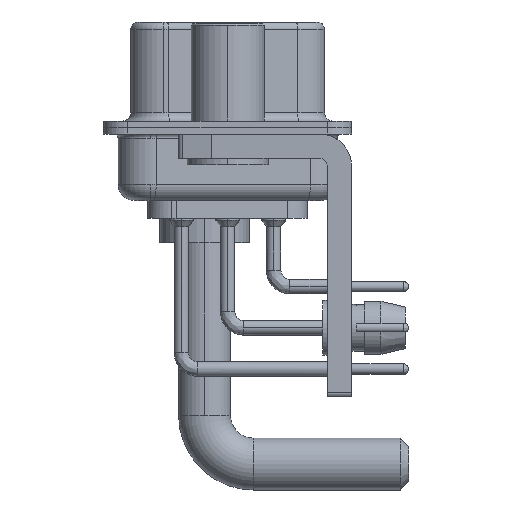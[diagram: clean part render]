
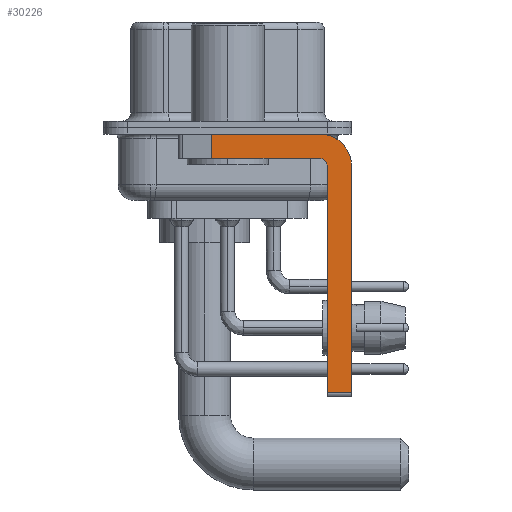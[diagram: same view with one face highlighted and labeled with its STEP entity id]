
A CAD part, left-side view. The second image highlights one B-rep face of the part: STEP entity #30226.
In plain terms, the highlighted planar face has unit normal (-1, 0, 0).
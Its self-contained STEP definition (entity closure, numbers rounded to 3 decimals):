
#754 = CIRCLE ( 'NONE', #32873, 2. ) ;
#1200 = DIRECTION ( 'NONE',  ( 0., -1., 0. ) ) ;
#2217 = AXIS2_PLACEMENT_3D ( 'NONE', #25078, #24886, #34525 ) ;
#3207 = VERTEX_POINT ( 'NONE', #11992 ) ;
#3504 = CIRCLE ( 'NONE', #2217, 0.5 ) ;
#3654 = CARTESIAN_POINT ( 'NONE',  ( -2.9, -6.15, -16.35 ) ) ;
#3787 = LINE ( 'NONE', #34758, #17340 ) ;
#4307 = VERTEX_POINT ( 'NONE', #29356 ) ;
#4416 = CARTESIAN_POINT ( 'NONE',  ( -2.9, -6.15, -2.4 ) ) ;
#4667 = VECTOR ( 'NONE', #13825, 1000. ) ;
#7042 = VERTEX_POINT ( 'NONE', #23971 ) ;
#7475 = ORIENTED_EDGE ( 'NONE', *, *, #37655, .F. ) ;
#8603 = DIRECTION ( 'NONE',  ( 0., 0., -1. ) ) ;
#8733 = CARTESIAN_POINT ( 'NONE',  ( -2.9, -5.65, -1.9 ) ) ;
#8794 = ORIENTED_EDGE ( 'NONE', *, *, #25865, .F. ) ;
#10162 = CARTESIAN_POINT ( 'NONE',  ( -2.9, -5.65, -0.4 ) ) ;
#11988 = ORIENTED_EDGE ( 'NONE', *, *, #27768, .F. ) ;
#11992 = CARTESIAN_POINT ( 'NONE',  ( -2.9, 0.978, -1.9 ) ) ;
#12527 = EDGE_CURVE ( 'NONE', #19139, #35585, #754, .T. ) ;
#12539 = VERTEX_POINT ( 'NONE', #3654 ) ;
#12830 = ORIENTED_EDGE ( 'NONE', *, *, #20391, .T. ) ;
#13825 = DIRECTION ( 'NONE',  ( 0., 1., 0. ) ) ;
#15504 = EDGE_CURVE ( 'NONE', #7042, #3207, #34600, .T. ) ;
#16035 = DIRECTION ( 'NONE',  ( 0., 0., -1. ) ) ;
#16162 = ORIENTED_EDGE ( 'NONE', *, *, #30370, .F. ) ;
#16312 = CARTESIAN_POINT ( 'NONE',  ( -2.9, -5.65, -2.4 ) ) ;
#16370 = VECTOR ( 'NONE', #39001, 1000. ) ;
#17340 = VECTOR ( 'NONE', #16035, 1000. ) ;
#17627 = AXIS2_PLACEMENT_3D ( 'NONE', #38975, #27314, #8603 ) ;
#17669 = DIRECTION ( 'NONE',  ( 0., -1., 0. ) ) ;
#17822 = LINE ( 'NONE', #30131, #29664 ) ;
#17860 = CARTESIAN_POINT ( 'NONE',  ( -2.9, 3., -0.4 ) ) ;
#18725 = ORIENTED_EDGE ( 'NONE', *, *, #15504, .T. ) ;
#19075 = VECTOR ( 'NONE', #1200, 1000. ) ;
#19139 = VERTEX_POINT ( 'NONE', #10162 ) ;
#20391 = EDGE_CURVE ( 'NONE', #12539, #4307, #31024, .T. ) ;
#21057 = FACE_OUTER_BOUND ( 'NONE', #24757, .T. ) ;
#22909 = CARTESIAN_POINT ( 'NONE',  ( -2.9, -5.65, -1.9 ) ) ;
#23730 = LINE ( 'NONE', #17860, #30975 ) ;
#23971 = CARTESIAN_POINT ( 'NONE',  ( -2.9, 0.978, -0.4 ) ) ;
#24103 = PLANE ( 'NONE',  #17627 ) ;
#24757 = EDGE_LOOP ( 'NONE', ( #11988, #18725, #7475, #16162, #8794, #12830, #38616, #29473 ) ) ;
#24886 = DIRECTION ( 'NONE',  ( -1., 0., 0. ) ) ;
#25078 = CARTESIAN_POINT ( 'NONE',  ( -2.9, -5.65, -2.4 ) ) ;
#25563 = CARTESIAN_POINT ( 'NONE',  ( -2.9, -7.65, -2.4 ) ) ;
#25865 = EDGE_CURVE ( 'NONE', #12539, #35719, #17822, .T. ) ;
#27306 = DIRECTION ( 'NONE',  ( 0., 0., 1. ) ) ;
#27314 = DIRECTION ( 'NONE',  ( 1., 0., 0. ) ) ;
#27768 = EDGE_CURVE ( 'NONE', #7042, #19139, #23730, .T. ) ;
#28514 = VERTEX_POINT ( 'NONE', #8733 ) ;
#29150 = LINE ( 'NONE', #22909, #4667 ) ;
#29356 = CARTESIAN_POINT ( 'NONE',  ( -2.9, -7.65, -16.35 ) ) ;
#29473 = ORIENTED_EDGE ( 'NONE', *, *, #12527, .F. ) ;
#29664 = VECTOR ( 'NONE', #27306, 1000. ) ;
#30131 = CARTESIAN_POINT ( 'NONE',  ( -2.9, -6.15, -16.6 ) ) ;
#30226 = ADVANCED_FACE ( 'NONE', ( #21057 ), #24103, .F. ) ;
#30370 = EDGE_CURVE ( 'NONE', #35719, #28514, #3504, .T. ) ;
#30975 = VECTOR ( 'NONE', #17669, 1000. ) ;
#31024 = LINE ( 'NONE', #37219, #19075 ) ;
#31239 = DIRECTION ( 'NONE',  ( 0., 0., -1. ) ) ;
#31595 = CARTESIAN_POINT ( 'NONE',  ( -2.9, 0.978, -1.9 ) ) ;
#32873 = AXIS2_PLACEMENT_3D ( 'NONE', #16312, #34236, #31239 ) ;
#34236 = DIRECTION ( 'NONE',  ( 1., 0., 0. ) ) ;
#34289 = EDGE_CURVE ( 'NONE', #35585, #4307, #3787, .T. ) ;
#34525 = DIRECTION ( 'NONE',  ( 0., 0., 1. ) ) ;
#34600 = LINE ( 'NONE', #31595, #16370 ) ;
#34758 = CARTESIAN_POINT ( 'NONE',  ( -2.9, -7.65, -2.4 ) ) ;
#35585 = VERTEX_POINT ( 'NONE', #25563 ) ;
#35719 = VERTEX_POINT ( 'NONE', #4416 ) ;
#37219 = CARTESIAN_POINT ( 'NONE',  ( -2.9, -5.65, -16.35 ) ) ;
#37655 = EDGE_CURVE ( 'NONE', #28514, #3207, #29150, .T. ) ;
#38616 = ORIENTED_EDGE ( 'NONE', *, *, #34289, .F. ) ;
#38975 = CARTESIAN_POINT ( 'NONE',  ( -2.9, -5.65, -2.4 ) ) ;
#39001 = DIRECTION ( 'NONE',  ( 0., 0., -1. ) ) ;
